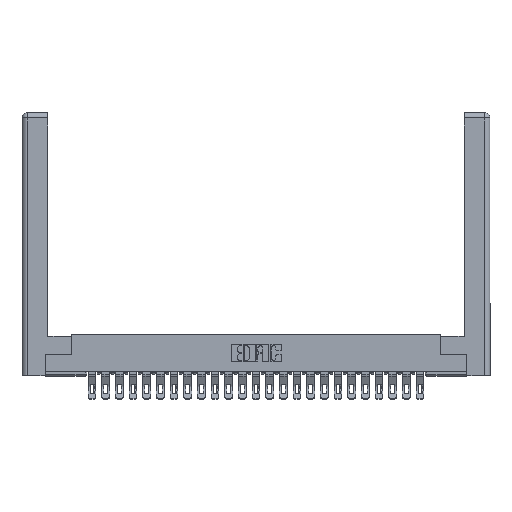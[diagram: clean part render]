
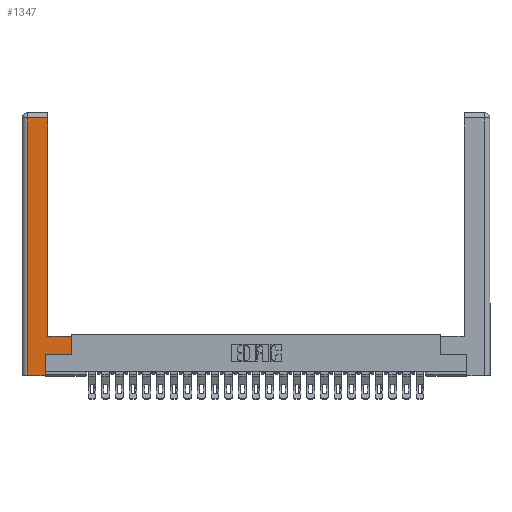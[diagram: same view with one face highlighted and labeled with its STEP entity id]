
A CAD part, top view. The second image highlights one B-rep face of the part: STEP entity #1347.
In plain terms, the highlighted planar face has unit normal (0, 0, 1).
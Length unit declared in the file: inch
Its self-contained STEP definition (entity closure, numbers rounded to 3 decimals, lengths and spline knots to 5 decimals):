
#573 = EDGE_CURVE ( 'NONE', #18030, #5252, #25647, .T. ) ;
#899 = DIRECTION ( 'NONE',  ( 0., 0., -1. ) ) ;
#1083 = EDGE_CURVE ( 'NONE', #16303, #24791, #26598, .T. ) ;
#1173 = VECTOR ( 'NONE', #14940, 39.37008 ) ;
#1347 = ADVANCED_FACE ( 'NONE', ( #20905 ), #26341, .F. ) ;
#1885 = DIRECTION ( 'NONE',  ( -1., 0., 0. ) ) ;
#1918 = DIRECTION ( 'NONE',  ( 1., 0., 0. ) ) ;
#2965 = CARTESIAN_POINT ( 'NONE',  ( 0.0615, 2.94, 0. ) ) ;
#2988 = VERTEX_POINT ( 'NONE', #13064 ) ;
#3977 = CARTESIAN_POINT ( 'NONE',  ( 0.565, 0.245, 0. ) ) ;
#4088 = EDGE_CURVE ( 'NONE', #24791, #19140, #21430, .T. ) ;
#4286 = CARTESIAN_POINT ( 'NONE',  ( 0.265, 0.245, 0. ) ) ;
#4438 = CARTESIAN_POINT ( 'NONE',  ( 0.265, 0., 0. ) ) ;
#5013 = LINE ( 'NONE', #14533, #14263 ) ;
#5252 = VERTEX_POINT ( 'NONE', #8561 ) ;
#5333 = ORIENTED_EDGE ( 'NONE', *, *, #22001, .T. ) ;
#6305 = CARTESIAN_POINT ( 'NONE',  ( 0.265, 0.245, 0. ) ) ;
#7836 = VERTEX_POINT ( 'NONE', #11145 ) ;
#8114 = LINE ( 'NONE', #26769, #18048 ) ;
#8324 = VECTOR ( 'NONE', #23485, 39.37008 ) ;
#8497 = CARTESIAN_POINT ( 'NONE',  ( 0.295, 3., 0. ) ) ;
#8561 = CARTESIAN_POINT ( 'NONE',  ( 0.565, 0.45, 0. ) ) ;
#10235 = VECTOR ( 'NONE', #26726, 39.37008 ) ;
#10716 = AXIS2_PLACEMENT_3D ( 'NONE', #13552, #899, #19987 ) ;
#11145 = CARTESIAN_POINT ( 'NONE',  ( 0.295, 2.94, 0. ) ) ;
#11754 = VECTOR ( 'NONE', #12746, 39.37008 ) ;
#11804 = EDGE_LOOP ( 'NONE', ( #5333, #22978, #15699, #27159, #12728, #26133, #17735, #27473 ) ) ;
#12728 = ORIENTED_EDGE ( 'NONE', *, *, #4088, .T. ) ;
#12746 = DIRECTION ( 'NONE',  ( 0., 1., 0. ) ) ;
#12754 = VECTOR ( 'NONE', #1918, 39.37008 ) ;
#12780 = EDGE_CURVE ( 'NONE', #19991, #16303, #25536, .T. ) ;
#13064 = CARTESIAN_POINT ( 'NONE',  ( 0.295, 0.45, 0. ) ) ;
#13552 = CARTESIAN_POINT ( 'NONE',  ( 0., 0., 0. ) ) ;
#13947 = EDGE_CURVE ( 'NONE', #19140, #18030, #22776, .T. ) ;
#14263 = VECTOR ( 'NONE', #1885, 39.37008 ) ;
#14415 = CARTESIAN_POINT ( 'NONE',  ( 0.0615, 0., 0. ) ) ;
#14533 = CARTESIAN_POINT ( 'NONE',  ( 0.295, 0.45, 0. ) ) ;
#14940 = DIRECTION ( 'NONE',  ( 0., 1., 0. ) ) ;
#15699 = ORIENTED_EDGE ( 'NONE', *, *, #12780, .T. ) ;
#16303 = VERTEX_POINT ( 'NONE', #20507 ) ;
#16412 = EDGE_CURVE ( 'NONE', #5252, #2988, #5013, .T. ) ;
#16498 = DIRECTION ( 'NONE',  ( -1., 0., 0. ) ) ;
#17735 = ORIENTED_EDGE ( 'NONE', *, *, #573, .T. ) ;
#18030 = VERTEX_POINT ( 'NONE', #3977 ) ;
#18048 = VECTOR ( 'NONE', #16498, 39.37008 ) ;
#19047 = LINE ( 'NONE', #8497, #1173 ) ;
#19140 = VERTEX_POINT ( 'NONE', #4286 ) ;
#19376 = DIRECTION ( 'NONE',  ( 0., 1., 0. ) ) ;
#19987 = DIRECTION ( 'NONE',  ( -1., 0., 0. ) ) ;
#19991 = VERTEX_POINT ( 'NONE', #2965 ) ;
#20507 = CARTESIAN_POINT ( 'NONE',  ( 0.0615, 0., 0. ) ) ;
#20905 = FACE_OUTER_BOUND ( 'NONE', #11804, .T. ) ;
#21430 = LINE ( 'NONE', #6305, #11754 ) ;
#22001 = EDGE_CURVE ( 'NONE', #2988, #7836, #19047, .T. ) ;
#22084 = CARTESIAN_POINT ( 'NONE',  ( 0.265, 0., 0. ) ) ;
#22298 = EDGE_CURVE ( 'NONE', #7836, #19991, #8114, .T. ) ;
#22776 = LINE ( 'NONE', #27359, #12754 ) ;
#22977 = VECTOR ( 'NONE', #19376, 39.37008 ) ;
#22978 = ORIENTED_EDGE ( 'NONE', *, *, #22298, .T. ) ;
#23485 = DIRECTION ( 'NONE',  ( 1., 0., 0. ) ) ;
#23612 = CARTESIAN_POINT ( 'NONE',  ( 0.565, 0.45, 0. ) ) ;
#24791 = VERTEX_POINT ( 'NONE', #22084 ) ;
#25536 = LINE ( 'NONE', #14415, #10235 ) ;
#25647 = LINE ( 'NONE', #23612, #22977 ) ;
#26133 = ORIENTED_EDGE ( 'NONE', *, *, #13947, .T. ) ;
#26341 = PLANE ( 'NONE',  #10716 ) ;
#26598 = LINE ( 'NONE', #4438, #8324 ) ;
#26726 = DIRECTION ( 'NONE',  ( 0., -1., 0. ) ) ;
#26769 = CARTESIAN_POINT ( 'NONE',  ( 0.0615, 2.94, 0. ) ) ;
#27159 = ORIENTED_EDGE ( 'NONE', *, *, #1083, .T. ) ;
#27359 = CARTESIAN_POINT ( 'NONE',  ( 0.565, 0.245, 0. ) ) ;
#27473 = ORIENTED_EDGE ( 'NONE', *, *, #16412, .T. ) ;
